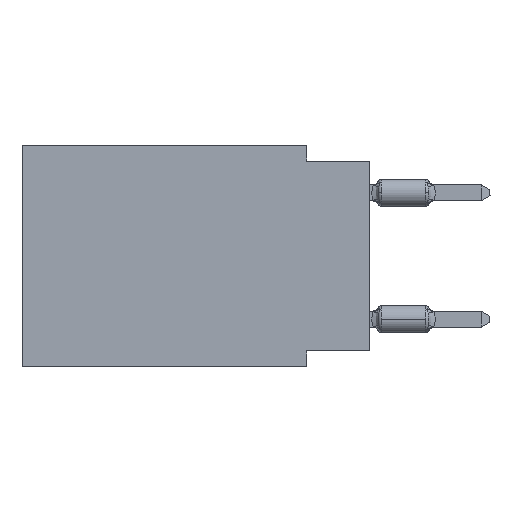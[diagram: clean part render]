
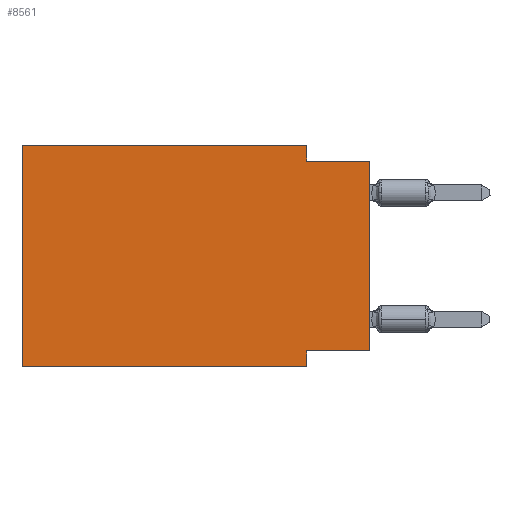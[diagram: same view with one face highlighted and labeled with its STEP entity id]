
A CAD part, left-side view. The second image highlights one B-rep face of the part: STEP entity #8561.
In plain terms, the highlighted planar face has unit normal (-1, 0, 0).
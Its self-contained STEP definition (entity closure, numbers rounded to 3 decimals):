
#85 = CARTESIAN_POINT ( 'NONE',  ( 0., 13.97, -8.89 ) ) ;
#399 = EDGE_CURVE ( 'NONE', #14018, #19569, #14560, .T. ) ;
#636 = CARTESIAN_POINT ( 'NONE',  ( 0., 13.97, 0. ) ) ;
#1402 = DIRECTION ( 'NONE',  ( 0., -1., 0. ) ) ;
#3622 = DIRECTION ( 'NONE',  ( 0., 0., 1. ) ) ;
#3828 = LINE ( 'NONE', #4008, #17104 ) ;
#4008 = CARTESIAN_POINT ( 'NONE',  ( 0., 0., -0.635 ) ) ;
#4056 = CARTESIAN_POINT ( 'NONE',  ( 0., 13.97, 0. ) ) ;
#4089 = EDGE_CURVE ( 'NONE', #34584, #35654, #20683, .T. ) ;
#4750 = CARTESIAN_POINT ( 'NONE',  ( 0., 0., -0.635 ) ) ;
#6035 = VERTEX_POINT ( 'NONE', #28414 ) ;
#6604 = CARTESIAN_POINT ( 'NONE',  ( 0., 2.54, -8.89 ) ) ;
#6658 = EDGE_LOOP ( 'NONE', ( #30879, #17751, #12428, #23773, #13725, #7630, #16015, #31680 ) ) ;
#6769 = VECTOR ( 'NONE', #3622, 1000. ) ;
#7630 = ORIENTED_EDGE ( 'NONE', *, *, #34731, .T. ) ;
#7844 = VERTEX_POINT ( 'NONE', #33238 ) ;
#8561 = ADVANCED_FACE ( 'NONE', ( #32605 ), #29819, .F. ) ;
#10608 = VERTEX_POINT ( 'NONE', #6604 ) ;
#11100 = VECTOR ( 'NONE', #17168, 1000. ) ;
#11147 = VECTOR ( 'NONE', #23103, 1000. ) ;
#12428 = ORIENTED_EDGE ( 'NONE', *, *, #19859, .F. ) ;
#12804 = EDGE_CURVE ( 'NONE', #7844, #10608, #31115, .T. ) ;
#13725 = ORIENTED_EDGE ( 'NONE', *, *, #35877, .F. ) ;
#14018 = VERTEX_POINT ( 'NONE', #21718 ) ;
#14209 = LINE ( 'NONE', #25888, #11147 ) ;
#14341 = VECTOR ( 'NONE', #29345, 1000. ) ;
#14560 = LINE ( 'NONE', #636, #30251 ) ;
#14925 = CARTESIAN_POINT ( 'NONE',  ( 0., 2.54, -0.635 ) ) ;
#15141 = EDGE_CURVE ( 'NONE', #18883, #35654, #3828, .T. ) ;
#15619 = CARTESIAN_POINT ( 'NONE',  ( 0., 0., -8.255 ) ) ;
#16015 = ORIENTED_EDGE ( 'NONE', *, *, #12804, .F. ) ;
#16070 = LINE ( 'NONE', #35162, #18436 ) ;
#17031 = DIRECTION ( 'NONE',  ( 0., 0., -1. ) ) ;
#17104 = VECTOR ( 'NONE', #1402, 1000. ) ;
#17168 = DIRECTION ( 'NONE',  ( 0., -1., 0. ) ) ;
#17751 = ORIENTED_EDGE ( 'NONE', *, *, #15141, .F. ) ;
#18436 = VECTOR ( 'NONE', #21096, 1000. ) ;
#18883 = VERTEX_POINT ( 'NONE', #14925 ) ;
#19569 = VERTEX_POINT ( 'NONE', #33574 ) ;
#19859 = EDGE_CURVE ( 'NONE', #19569, #18883, #16070, .T. ) ;
#19987 = CARTESIAN_POINT ( 'NONE',  ( 0., 2.54, -8.89 ) ) ;
#20683 = LINE ( 'NONE', #34755, #6769 ) ;
#20734 = EDGE_CURVE ( 'NONE', #34584, #7844, #30064, .T. ) ;
#21096 = DIRECTION ( 'NONE',  ( 0., 0., -1. ) ) ;
#21100 = VECTOR ( 'NONE', #17031, 1000. ) ;
#21718 = CARTESIAN_POINT ( 'NONE',  ( 0., 13.97, 0. ) ) ;
#23103 = DIRECTION ( 'NONE',  ( 0., 0., 1. ) ) ;
#23348 = DIRECTION ( 'NONE',  ( 0., 0., -1. ) ) ;
#23773 = ORIENTED_EDGE ( 'NONE', *, *, #399, .F. ) ;
#25519 = LINE ( 'NONE', #85, #11100 ) ;
#25888 = CARTESIAN_POINT ( 'NONE',  ( 0., 13.97, 0. ) ) ;
#28414 = CARTESIAN_POINT ( 'NONE',  ( 0., 13.97, -8.89 ) ) ;
#29345 = DIRECTION ( 'NONE',  ( 0., 1., 0. ) ) ;
#29819 = PLANE ( 'NONE',  #32978 ) ;
#30064 = LINE ( 'NONE', #15619, #14341 ) ;
#30251 = VECTOR ( 'NONE', #31608, 1000. ) ;
#30879 = ORIENTED_EDGE ( 'NONE', *, *, #4089, .T. ) ;
#31115 = LINE ( 'NONE', #19987, #21100 ) ;
#31608 = DIRECTION ( 'NONE',  ( 0., -1., 0. ) ) ;
#31680 = ORIENTED_EDGE ( 'NONE', *, *, #20734, .F. ) ;
#32053 = DIRECTION ( 'NONE',  ( 1., 0., 0. ) ) ;
#32605 = FACE_OUTER_BOUND ( 'NONE', #6658, .T. ) ;
#32978 = AXIS2_PLACEMENT_3D ( 'NONE', #4056, #32053, #23348 ) ;
#33114 = CARTESIAN_POINT ( 'NONE',  ( 0., 0., -8.255 ) ) ;
#33238 = CARTESIAN_POINT ( 'NONE',  ( 0., 2.54, -8.255 ) ) ;
#33574 = CARTESIAN_POINT ( 'NONE',  ( 0., 2.54, 0. ) ) ;
#34584 = VERTEX_POINT ( 'NONE', #33114 ) ;
#34731 = EDGE_CURVE ( 'NONE', #6035, #10608, #25519, .T. ) ;
#34755 = CARTESIAN_POINT ( 'NONE',  ( 0., 0., 0. ) ) ;
#35162 = CARTESIAN_POINT ( 'NONE',  ( 0., 2.54, 0. ) ) ;
#35654 = VERTEX_POINT ( 'NONE', #4750 ) ;
#35877 = EDGE_CURVE ( 'NONE', #6035, #14018, #14209, .T. ) ;
